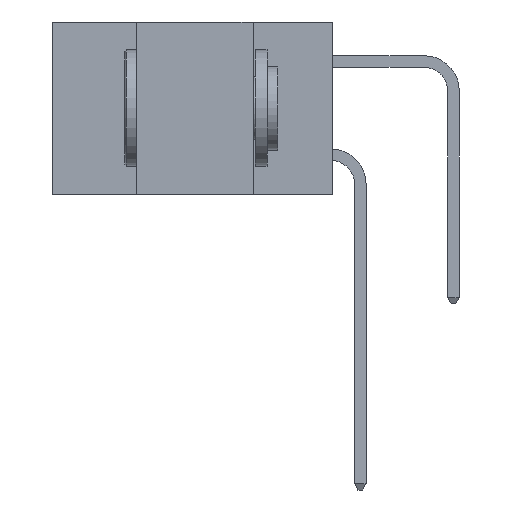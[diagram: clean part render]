
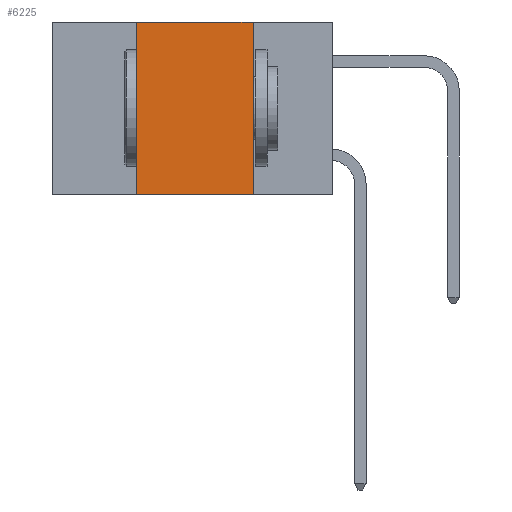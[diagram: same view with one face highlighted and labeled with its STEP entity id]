
A CAD part, left-side view. The second image highlights one B-rep face of the part: STEP entity #6225.
In plain terms, the highlighted planar face has unit normal (-1, 0, 0).
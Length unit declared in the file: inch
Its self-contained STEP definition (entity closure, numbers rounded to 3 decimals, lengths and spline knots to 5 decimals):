
#523 = ORIENTED_EDGE ( 'NONE', *, *, #10700, .F. ) ;
#752 = CARTESIAN_POINT ( 'NONE',  ( 0., 0.17, -0.37 ) ) ;
#1224 = CARTESIAN_POINT ( 'NONE',  ( 0., 0.17, -0.37 ) ) ;
#1252 = LINE ( 'NONE', #6382, #18583 ) ;
#2801 = ORIENTED_EDGE ( 'NONE', *, *, #4864, .T. ) ;
#2994 = DIRECTION ( 'NONE',  ( 0., 0., -1. ) ) ;
#4277 = LINE ( 'NONE', #22173, #9387 ) ;
#4285 = ORIENTED_EDGE ( 'NONE', *, *, #6327, .F. ) ;
#4864 = EDGE_CURVE ( 'NONE', #19717, #27685, #1252, .T. ) ;
#5796 = EDGE_LOOP ( 'NONE', ( #523, #6281, #4285, #2801 ) ) ;
#6046 = DIRECTION ( 'NONE',  ( 0., -1., 0. ) ) ;
#6225 = ADVANCED_FACE ( 'NONE', ( #7000 ), #24650, .F. ) ;
#6281 = ORIENTED_EDGE ( 'NONE', *, *, #9242, .F. ) ;
#6327 = EDGE_CURVE ( 'NONE', #19717, #17572, #4277, .T. ) ;
#6382 = CARTESIAN_POINT ( 'NONE',  ( 0., 0.6, -0.37 ) ) ;
#7000 = FACE_OUTER_BOUND ( 'NONE', #5796, .T. ) ;
#8388 = CARTESIAN_POINT ( 'NONE',  ( 0., 0.42, 0. ) ) ;
#9242 = EDGE_CURVE ( 'NONE', #17572, #14100, #10916, .T. ) ;
#9387 = VECTOR ( 'NONE', #22253, 39.37008 ) ;
#9846 = LINE ( 'NONE', #752, #19960 ) ;
#10080 = CARTESIAN_POINT ( 'NONE',  ( 0., 0.17, 0. ) ) ;
#10700 = EDGE_CURVE ( 'NONE', #14100, #27685, #9846, .T. ) ;
#10916 = LINE ( 'NONE', #14499, #16662 ) ;
#14100 = VERTEX_POINT ( 'NONE', #10080 ) ;
#14499 = CARTESIAN_POINT ( 'NONE',  ( 0., 0.6, 0. ) ) ;
#15187 = DIRECTION ( 'NONE',  ( 0., -1., 0. ) ) ;
#16662 = VECTOR ( 'NONE', #15187, 39.37008 ) ;
#17572 = VERTEX_POINT ( 'NONE', #8388 ) ;
#18583 = VECTOR ( 'NONE', #6046, 39.37008 ) ;
#19510 = CARTESIAN_POINT ( 'NONE',  ( 0., 0.42, -0.37 ) ) ;
#19717 = VERTEX_POINT ( 'NONE', #19510 ) ;
#19960 = VECTOR ( 'NONE', #2994, 39.37008 ) ;
#22173 = CARTESIAN_POINT ( 'NONE',  ( 0., 0.42, -0.37 ) ) ;
#22253 = DIRECTION ( 'NONE',  ( 0., 0., 1. ) ) ;
#23979 = DIRECTION ( 'NONE',  ( 0., 0., -1. ) ) ;
#24006 = DIRECTION ( 'NONE',  ( 1., 0., 0. ) ) ;
#24650 = PLANE ( 'NONE',  #27815 ) ;
#24814 = CARTESIAN_POINT ( 'NONE',  ( 0., 0.6, 0. ) ) ;
#27685 = VERTEX_POINT ( 'NONE', #1224 ) ;
#27815 = AXIS2_PLACEMENT_3D ( 'NONE', #24814, #24006, #23979 ) ;
